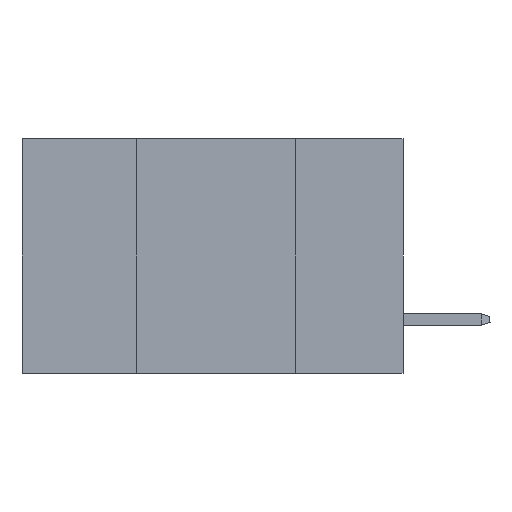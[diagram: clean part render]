
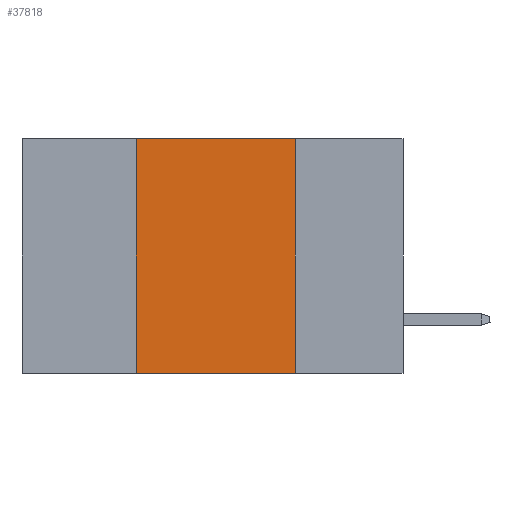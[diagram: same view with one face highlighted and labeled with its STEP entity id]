
A CAD part, left-side view. The second image highlights one B-rep face of the part: STEP entity #37818.
In plain terms, the highlighted planar face has unit normal (-1, 0, 0).
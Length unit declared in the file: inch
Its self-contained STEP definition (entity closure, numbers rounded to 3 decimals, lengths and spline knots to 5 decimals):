
#148 = VECTOR ( 'NONE', #15049, 39.37008 ) ;
#2890 = ORIENTED_EDGE ( 'NONE', *, *, #7765, .F. ) ;
#3995 = ORIENTED_EDGE ( 'NONE', *, *, #27026, .T. ) ;
#4499 = CARTESIAN_POINT ( 'NONE',  ( 0., 0.6, 0. ) ) ;
#4502 = LINE ( 'NONE', #11131, #26480 ) ;
#4558 = DIRECTION ( 'NONE',  ( 0., 0., 1. ) ) ;
#4783 = CARTESIAN_POINT ( 'NONE',  ( 0., 0.6, -0.37 ) ) ;
#7066 = CARTESIAN_POINT ( 'NONE',  ( 0., 0.17, 0. ) ) ;
#7277 = DIRECTION ( 'NONE',  ( 0., 0., -1. ) ) ;
#7315 = EDGE_LOOP ( 'NONE', ( #38887, #2890, #30580, #3995 ) ) ;
#7756 = CARTESIAN_POINT ( 'NONE',  ( 0., 0.42, 0. ) ) ;
#7765 = EDGE_CURVE ( 'NONE', #26354, #18148, #4502, .T. ) ;
#9101 = CARTESIAN_POINT ( 'NONE',  ( 0., 0.17, 0. ) ) ;
#11131 = CARTESIAN_POINT ( 'NONE',  ( 0., 0.6, 0. ) ) ;
#11761 = DIRECTION ( 'NONE',  ( 0., 0., -1. ) ) ;
#14076 = VECTOR ( 'NONE', #7277, 39.37008 ) ;
#14841 = LINE ( 'NONE', #4783, #148 ) ;
#15049 = DIRECTION ( 'NONE',  ( 0., -1., 0. ) ) ;
#18039 = AXIS2_PLACEMENT_3D ( 'NONE', #4499, #18184, #11761 ) ;
#18148 = VERTEX_POINT ( 'NONE', #9101 ) ;
#18184 = DIRECTION ( 'NONE',  ( 1., 0., 0. ) ) ;
#18186 = DIRECTION ( 'NONE',  ( 0., -1., 0. ) ) ;
#19893 = CARTESIAN_POINT ( 'NONE',  ( 0., 0.17, -0.37 ) ) ;
#26354 = VERTEX_POINT ( 'NONE', #33078 ) ;
#26480 = VECTOR ( 'NONE', #18186, 39.37008 ) ;
#27026 = EDGE_CURVE ( 'NONE', #29297, #30779, #14841, .T. ) ;
#27371 = PLANE ( 'NONE',  #18039 ) ;
#29297 = VERTEX_POINT ( 'NONE', #35462 ) ;
#30580 = ORIENTED_EDGE ( 'NONE', *, *, #42025, .F. ) ;
#30779 = VERTEX_POINT ( 'NONE', #19893 ) ;
#31209 = FACE_OUTER_BOUND ( 'NONE', #7315, .T. ) ;
#32522 = VECTOR ( 'NONE', #4558, 39.37008 ) ;
#33078 = CARTESIAN_POINT ( 'NONE',  ( 0., 0.42, 0. ) ) ;
#35462 = CARTESIAN_POINT ( 'NONE',  ( 0., 0.42, -0.37 ) ) ;
#37061 = LINE ( 'NONE', #7756, #32522 ) ;
#37818 = ADVANCED_FACE ( 'NONE', ( #31209 ), #27371, .F. ) ;
#38887 = ORIENTED_EDGE ( 'NONE', *, *, #39811, .F. ) ;
#39811 = EDGE_CURVE ( 'NONE', #18148, #30779, #41195, .T. ) ;
#41195 = LINE ( 'NONE', #7066, #14076 ) ;
#42025 = EDGE_CURVE ( 'NONE', #29297, #26354, #37061, .T. ) ;
